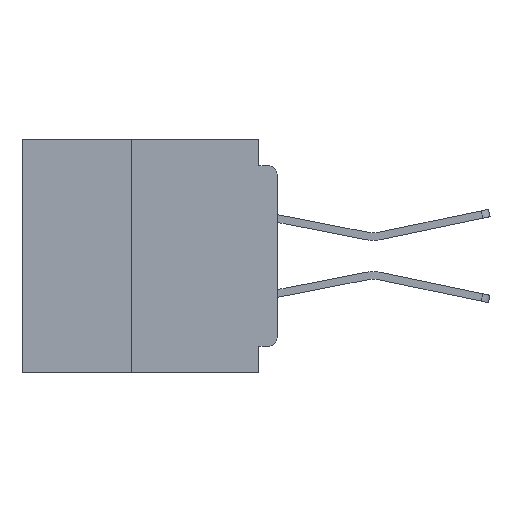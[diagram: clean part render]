
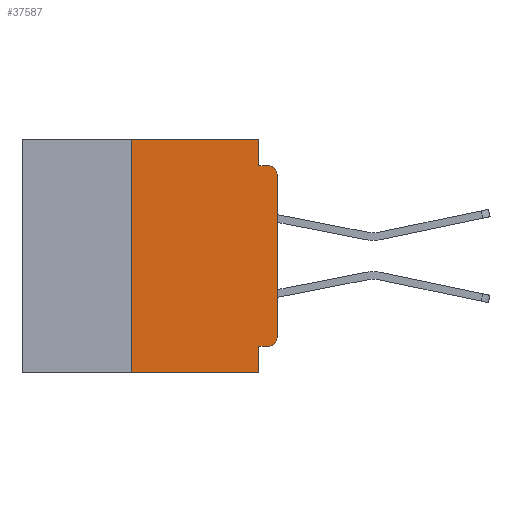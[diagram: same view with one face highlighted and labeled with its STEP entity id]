
A CAD part, left-side view. The second image highlights one B-rep face of the part: STEP entity #37587.
In plain terms, the highlighted planar face has unit normal (-1, 0, 0).
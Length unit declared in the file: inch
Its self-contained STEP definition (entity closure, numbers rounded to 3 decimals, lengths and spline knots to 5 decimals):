
#643 = VECTOR ( 'NONE', #21858, 39.37008 ) ;
#1159 = ORIENTED_EDGE ( 'NONE', *, *, #22001, .T. ) ;
#1257 = CARTESIAN_POINT ( 'NONE',  ( 0., 0., -0.045 ) ) ;
#1557 = ORIENTED_EDGE ( 'NONE', *, *, #23669, .T. ) ;
#1939 = AXIS2_PLACEMENT_3D ( 'NONE', #28746, #10236, #31887 ) ;
#2614 = ORIENTED_EDGE ( 'NONE', *, *, #7914, .T. ) ;
#2784 = VECTOR ( 'NONE', #9509, 39.37008 ) ;
#3036 = PLANE ( 'NONE',  #22609 ) ;
#4120 = VERTEX_POINT ( 'NONE', #31612 ) ;
#4307 = CARTESIAN_POINT ( 'NONE',  ( 0., 0.031, -0.4 ) ) ;
#4589 = EDGE_CURVE ( 'NONE', #13239, #4120, #29489, .T. ) ;
#4820 = EDGE_CURVE ( 'NONE', #19691, #28412, #6197, .T. ) ;
#5438 = CARTESIAN_POINT ( 'NONE',  ( 0., 0., 0. ) ) ;
#5619 = VERTEX_POINT ( 'NONE', #36379 ) ;
#6197 = LINE ( 'NONE', #1257, #27975 ) ;
#6365 = CARTESIAN_POINT ( 'NONE',  ( 0., 0., -0.355 ) ) ;
#7186 = VERTEX_POINT ( 'NONE', #23487 ) ;
#7840 = EDGE_LOOP ( 'NONE', ( #2614, #35117, #14821, #14879, #16211, #20764, #1557, #15773, #12172, #1159 ) ) ;
#7914 = EDGE_CURVE ( 'NONE', #10807, #14910, #21630, .T. ) ;
#8067 = LINE ( 'NONE', #31962, #33696 ) ;
#8413 = CARTESIAN_POINT ( 'NONE',  ( 0., 0., -0.34 ) ) ;
#8943 = CARTESIAN_POINT ( 'NONE',  ( 0., 0., -0.06 ) ) ;
#9466 = DIRECTION ( 'NONE',  ( 0., 0., -1. ) ) ;
#9509 = DIRECTION ( 'NONE',  ( 0., 1., 0. ) ) ;
#9717 = CIRCLE ( 'NONE', #12512, 0.015 ) ;
#10236 = DIRECTION ( 'NONE',  ( -1., 0., 0. ) ) ;
#10807 = VERTEX_POINT ( 'NONE', #8413 ) ;
#11441 = DIRECTION ( 'NONE',  ( -1., 0., 0. ) ) ;
#11700 = DIRECTION ( 'NONE',  ( 0., 0., 1. ) ) ;
#11866 = CARTESIAN_POINT ( 'NONE',  ( 0., 0.031, 0. ) ) ;
#12172 = ORIENTED_EDGE ( 'NONE', *, *, #4589, .F. ) ;
#12512 = AXIS2_PLACEMENT_3D ( 'NONE', #29948, #11441, #33091 ) ;
#13239 = VERTEX_POINT ( 'NONE', #17120 ) ;
#13419 = DIRECTION ( 'NONE',  ( 0., -1., 0. ) ) ;
#13470 = VECTOR ( 'NONE', #11700, 39.37008 ) ;
#14821 = ORIENTED_EDGE ( 'NONE', *, *, #4820, .F. ) ;
#14879 = ORIENTED_EDGE ( 'NONE', *, *, #24002, .F. ) ;
#14910 = VERTEX_POINT ( 'NONE', #8943 ) ;
#15557 = CARTESIAN_POINT ( 'NONE',  ( 0., 0.437, 0. ) ) ;
#15725 = CARTESIAN_POINT ( 'NONE',  ( 0., 0.015, -0.045 ) ) ;
#15773 = ORIENTED_EDGE ( 'NONE', *, *, #23724, .F. ) ;
#16211 = ORIENTED_EDGE ( 'NONE', *, *, #32591, .F. ) ;
#16800 = DIRECTION ( 'NONE',  ( 0., -1., 0. ) ) ;
#16864 = CIRCLE ( 'NONE', #1939, 0.015 ) ;
#17120 = CARTESIAN_POINT ( 'NONE',  ( 0., 0.015, -0.355 ) ) ;
#17646 = EDGE_CURVE ( 'NONE', #5619, #7186, #32777, .T. ) ;
#17681 = VECTOR ( 'NONE', #35092, 39.37008 ) ;
#17882 = DIRECTION ( 'NONE',  ( 0., 0., -1. ) ) ;
#19691 = VERTEX_POINT ( 'NONE', #26036 ) ;
#20764 = ORIENTED_EDGE ( 'NONE', *, *, #17646, .F. ) ;
#21630 = LINE ( 'NONE', #5438, #13470 ) ;
#21858 = DIRECTION ( 'NONE',  ( 0., 0., 1. ) ) ;
#22001 = EDGE_CURVE ( 'NONE', #13239, #10807, #16864, .T. ) ;
#22609 = AXIS2_PLACEMENT_3D ( 'NONE', #15557, #27956, #9466 ) ;
#23487 = CARTESIAN_POINT ( 'NONE',  ( 0., 0.25, 0. ) ) ;
#23669 = EDGE_CURVE ( 'NONE', #5619, #28485, #28820, .T. ) ;
#23724 = EDGE_CURVE ( 'NONE', #4120, #28485, #29795, .T. ) ;
#24002 = EDGE_CURVE ( 'NONE', #29722, #19691, #33622, .T. ) ;
#25450 = CARTESIAN_POINT ( 'NONE',  ( 0., 0.437, -0.4 ) ) ;
#26036 = CARTESIAN_POINT ( 'NONE',  ( 0., 0.031, -0.045 ) ) ;
#26782 = FACE_OUTER_BOUND ( 'NONE', #7840, .T. ) ;
#27956 = DIRECTION ( 'NONE',  ( 1., 0., 0. ) ) ;
#27975 = VECTOR ( 'NONE', #16800, 39.37008 ) ;
#28084 = CARTESIAN_POINT ( 'NONE',  ( 0., 0.25, -0.4 ) ) ;
#28412 = VERTEX_POINT ( 'NONE', #15725 ) ;
#28485 = VERTEX_POINT ( 'NONE', #4307 ) ;
#28746 = CARTESIAN_POINT ( 'NONE',  ( 0., 0.015, -0.34 ) ) ;
#28820 = LINE ( 'NONE', #25450, #36111 ) ;
#29489 = LINE ( 'NONE', #6365, #2784 ) ;
#29722 = VERTEX_POINT ( 'NONE', #11866 ) ;
#29795 = LINE ( 'NONE', #32009, #17681 ) ;
#29948 = CARTESIAN_POINT ( 'NONE',  ( 0., 0.015, -0.06 ) ) ;
#31612 = CARTESIAN_POINT ( 'NONE',  ( 0., 0.031, -0.355 ) ) ;
#31724 = VECTOR ( 'NONE', #17882, 39.37008 ) ;
#31734 = DIRECTION ( 'NONE',  ( 0., -1., 0. ) ) ;
#31887 = DIRECTION ( 'NONE',  ( 0., 0., -1. ) ) ;
#31962 = CARTESIAN_POINT ( 'NONE',  ( 0., 0.437, 0. ) ) ;
#32009 = CARTESIAN_POINT ( 'NONE',  ( 0., 0.031, -0.4 ) ) ;
#32591 = EDGE_CURVE ( 'NONE', #7186, #29722, #8067, .T. ) ;
#32777 = LINE ( 'NONE', #28084, #643 ) ;
#33091 = DIRECTION ( 'NONE',  ( 0., 0., -1. ) ) ;
#33622 = LINE ( 'NONE', #36450, #31724 ) ;
#33696 = VECTOR ( 'NONE', #13419, 39.37008 ) ;
#35092 = DIRECTION ( 'NONE',  ( 0., 0., -1. ) ) ;
#35117 = ORIENTED_EDGE ( 'NONE', *, *, #36696, .T. ) ;
#36111 = VECTOR ( 'NONE', #31734, 39.37008 ) ;
#36379 = CARTESIAN_POINT ( 'NONE',  ( 0., 0.25, -0.4 ) ) ;
#36450 = CARTESIAN_POINT ( 'NONE',  ( 0., 0.031, 0. ) ) ;
#36696 = EDGE_CURVE ( 'NONE', #14910, #28412, #9717, .T. ) ;
#37587 = ADVANCED_FACE ( 'NONE', ( #26782 ), #3036, .F. ) ;
